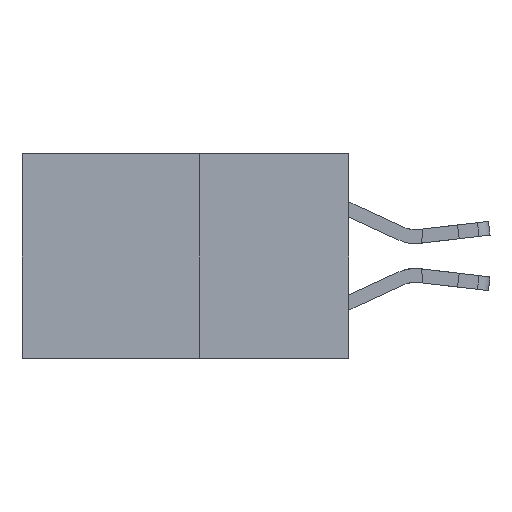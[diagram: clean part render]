
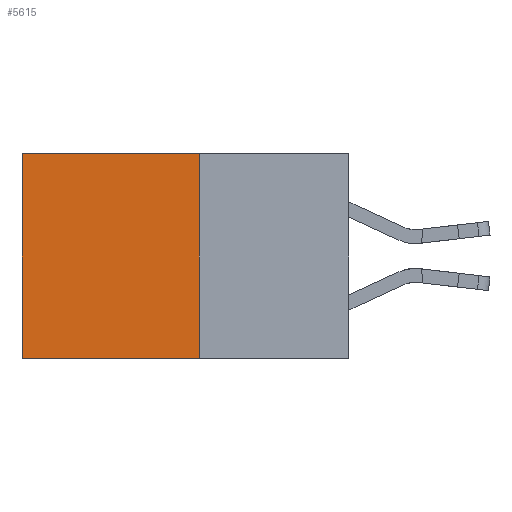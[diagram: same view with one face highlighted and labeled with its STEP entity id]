
A CAD part, left-side view. The second image highlights one B-rep face of the part: STEP entity #5615.
In plain terms, the highlighted planar face has unit normal (-1, 0, 0).
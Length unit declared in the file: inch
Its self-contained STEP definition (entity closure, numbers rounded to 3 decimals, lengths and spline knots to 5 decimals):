
#1489 = VERTEX_POINT ( 'NONE', #29401 ) ;
#1615 = DIRECTION ( 'NONE',  ( 0., 0., -1. ) ) ;
#2301 = PLANE ( 'NONE',  #11930 ) ;
#4614 = DIRECTION ( 'NONE',  ( 1., 0., 0. ) ) ;
#5081 = CARTESIAN_POINT ( 'NONE',  ( 0.277, 0.27, -0.37 ) ) ;
#5615 = ADVANCED_FACE ( 'NONE', ( #8531 ), #2301, .F. ) ;
#5716 = CARTESIAN_POINT ( 'NONE',  ( 0.277, 0.59, -0.37 ) ) ;
#7389 = DIRECTION ( 'NONE',  ( 0., 1., 0. ) ) ;
#7410 = LINE ( 'NONE', #21432, #12729 ) ;
#7777 = DIRECTION ( 'NONE',  ( 0., 1., 0. ) ) ;
#7861 = EDGE_CURVE ( 'NONE', #19542, #1489, #7410, .T. ) ;
#8531 = FACE_OUTER_BOUND ( 'NONE', #29342, .T. ) ;
#8915 = VECTOR ( 'NONE', #1615, 39.37008 ) ;
#9286 = ORIENTED_EDGE ( 'NONE', *, *, #18840, .T. ) ;
#11930 = AXIS2_PLACEMENT_3D ( 'NONE', #18236, #4614, #20536 ) ;
#12033 = VECTOR ( 'NONE', #7389, 39.37008 ) ;
#12729 = VECTOR ( 'NONE', #7777, 39.37008 ) ;
#12754 = LINE ( 'NONE', #23329, #12033 ) ;
#13002 = CARTESIAN_POINT ( 'NONE',  ( 0.277, 0.27, -0.37 ) ) ;
#14028 = VERTEX_POINT ( 'NONE', #22004 ) ;
#16479 = LINE ( 'NONE', #5716, #24319 ) ;
#16635 = EDGE_CURVE ( 'NONE', #14028, #19542, #21060, .T. ) ;
#16671 = ORIENTED_EDGE ( 'NONE', *, *, #16635, .F. ) ;
#18236 = CARTESIAN_POINT ( 'NONE',  ( 0.277, 0.27, -0.37 ) ) ;
#18840 = EDGE_CURVE ( 'NONE', #14028, #27505, #12754, .T. ) ;
#19542 = VERTEX_POINT ( 'NONE', #5081 ) ;
#20536 = DIRECTION ( 'NONE',  ( 0., 0., -1. ) ) ;
#21060 = LINE ( 'NONE', #13002, #8915 ) ;
#21432 = CARTESIAN_POINT ( 'NONE',  ( 0.277, 0.27, -0.37 ) ) ;
#21627 = DIRECTION ( 'NONE',  ( 0., 0., -1. ) ) ;
#22004 = CARTESIAN_POINT ( 'NONE',  ( 0.277, 0.27, 0. ) ) ;
#22231 = ORIENTED_EDGE ( 'NONE', *, *, #7861, .F. ) ;
#22251 = EDGE_CURVE ( 'NONE', #27505, #1489, #16479, .T. ) ;
#23329 = CARTESIAN_POINT ( 'NONE',  ( 0.277, 0.27, 0. ) ) ;
#24319 = VECTOR ( 'NONE', #21627, 39.37008 ) ;
#26336 = CARTESIAN_POINT ( 'NONE',  ( 0.277, 0.59, 0. ) ) ;
#27505 = VERTEX_POINT ( 'NONE', #26336 ) ;
#29080 = ORIENTED_EDGE ( 'NONE', *, *, #22251, .T. ) ;
#29342 = EDGE_LOOP ( 'NONE', ( #29080, #22231, #16671, #9286 ) ) ;
#29401 = CARTESIAN_POINT ( 'NONE',  ( 0.277, 0.59, -0.37 ) ) ;
